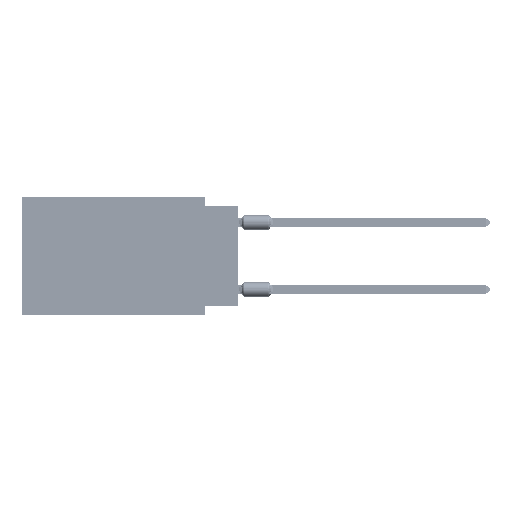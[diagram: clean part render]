
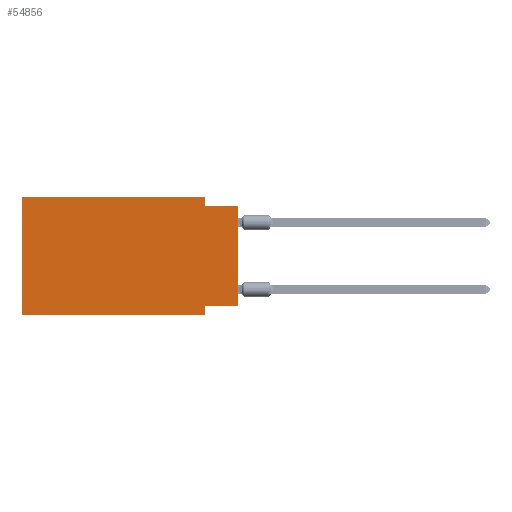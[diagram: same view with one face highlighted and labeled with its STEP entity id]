
A CAD part, left-side view. The second image highlights one B-rep face of the part: STEP entity #54856.
In plain terms, the highlighted planar face has unit normal (-1, 0, 0).
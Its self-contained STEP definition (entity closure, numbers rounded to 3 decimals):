
#1090 = VERTEX_POINT ( 'NONE', #2675 ) ;
#2675 = CARTESIAN_POINT ( 'NONE',  ( 0., 0., -0.635 ) ) ;
#5478 = EDGE_CURVE ( 'NONE', #78072, #86464, #22740, .T. ) ;
#10530 = LINE ( 'NONE', #24280, #24152 ) ;
#12280 = DIRECTION ( 'NONE',  ( 0., 0., -1. ) ) ;
#12432 = PLANE ( 'NONE',  #39319 ) ;
#13697 = CARTESIAN_POINT ( 'NONE',  ( 0., 16.383, 0. ) ) ;
#14303 = EDGE_LOOP ( 'NONE', ( #94507, #85639, #62938, #16057, #21806, #57369, #17778, #51122 ) ) ;
#15489 = LINE ( 'NONE', #13697, #29186 ) ;
#16057 = ORIENTED_EDGE ( 'NONE', *, *, #51140, .F. ) ;
#16251 = CARTESIAN_POINT ( 'NONE',  ( 0., 2.54, -8.89 ) ) ;
#17050 = VECTOR ( 'NONE', #87482, 1000. ) ;
#17396 = CARTESIAN_POINT ( 'NONE',  ( 0., 16.383, -8.89 ) ) ;
#17778 = ORIENTED_EDGE ( 'NONE', *, *, #53410, .F. ) ;
#19549 = CARTESIAN_POINT ( 'NONE',  ( 0., 0., -8.255 ) ) ;
#20548 = VERTEX_POINT ( 'NONE', #93034 ) ;
#21164 = VERTEX_POINT ( 'NONE', #45767 ) ;
#21294 = CARTESIAN_POINT ( 'NONE',  ( 0., 16.383, 0. ) ) ;
#21304 = VECTOR ( 'NONE', #44368, 1000. ) ;
#21806 = ORIENTED_EDGE ( 'NONE', *, *, #5478, .F. ) ;
#22740 = LINE ( 'NONE', #21294, #21304 ) ;
#23143 = LINE ( 'NONE', #16251, #23464 ) ;
#23371 = CARTESIAN_POINT ( 'NONE',  ( 0., 0., -8.255 ) ) ;
#23464 = VECTOR ( 'NONE', #46205, 1000. ) ;
#24152 = VECTOR ( 'NONE', #40495, 1000. ) ;
#24280 = CARTESIAN_POINT ( 'NONE',  ( 0., 0., -0.635 ) ) ;
#25070 = LINE ( 'NONE', #85892, #81074 ) ;
#26022 = VECTOR ( 'NONE', #60799, 1000. ) ;
#26183 = DIRECTION ( 'NONE',  ( 1., 0., 0. ) ) ;
#26671 = DIRECTION ( 'NONE',  ( 0., 0., -1. ) ) ;
#29186 = VECTOR ( 'NONE', #35810, 1000. ) ;
#30837 = EDGE_CURVE ( 'NONE', #20548, #40981, #25070, .T. ) ;
#30853 = LINE ( 'NONE', #68627, #26022 ) ;
#31226 = DIRECTION ( 'NONE',  ( 0., 1., 0. ) ) ;
#35810 = DIRECTION ( 'NONE',  ( 0., -1., 0. ) ) ;
#39168 = VERTEX_POINT ( 'NONE', #55024 ) ;
#39319 = AXIS2_PLACEMENT_3D ( 'NONE', #49263, #26183, #26671 ) ;
#39852 = EDGE_CURVE ( 'NONE', #67837, #21164, #74428, .T. ) ;
#40495 = DIRECTION ( 'NONE',  ( 0., -1., 0. ) ) ;
#40561 = VECTOR ( 'NONE', #31226, 1000. ) ;
#40981 = VERTEX_POINT ( 'NONE', #73010 ) ;
#41421 = FACE_OUTER_BOUND ( 'NONE', #14303, .T. ) ;
#41853 = EDGE_CURVE ( 'NONE', #78072, #39168, #72787, .T. ) ;
#44368 = DIRECTION ( 'NONE',  ( 0., 0., 1. ) ) ;
#45767 = CARTESIAN_POINT ( 'NONE',  ( 0., 2.54, -8.255 ) ) ;
#46205 = DIRECTION ( 'NONE',  ( 0., 0., -1. ) ) ;
#49263 = CARTESIAN_POINT ( 'NONE',  ( 0., 16.383, 0. ) ) ;
#51122 = ORIENTED_EDGE ( 'NONE', *, *, #39852, .F. ) ;
#51140 = EDGE_CURVE ( 'NONE', #86464, #20548, #15489, .T. ) ;
#53410 = EDGE_CURVE ( 'NONE', #21164, #39168, #23143, .T. ) ;
#54856 = ADVANCED_FACE ( 'NONE', ( #41421 ), #12432, .F. ) ;
#55024 = CARTESIAN_POINT ( 'NONE',  ( 0., 2.54, -8.89 ) ) ;
#57369 = ORIENTED_EDGE ( 'NONE', *, *, #41853, .T. ) ;
#60799 = DIRECTION ( 'NONE',  ( 0., 0., 1. ) ) ;
#62938 = ORIENTED_EDGE ( 'NONE', *, *, #30837, .F. ) ;
#67837 = VERTEX_POINT ( 'NONE', #19549 ) ;
#68580 = CARTESIAN_POINT ( 'NONE',  ( 0., 16.383, 0. ) ) ;
#68627 = CARTESIAN_POINT ( 'NONE',  ( 0., 0., 0. ) ) ;
#72787 = LINE ( 'NONE', #93861, #17050 ) ;
#73010 = CARTESIAN_POINT ( 'NONE',  ( 0., 2.54, -0.635 ) ) ;
#74428 = LINE ( 'NONE', #23371, #40561 ) ;
#77844 = EDGE_CURVE ( 'NONE', #67837, #1090, #30853, .T. ) ;
#78072 = VERTEX_POINT ( 'NONE', #17396 ) ;
#81074 = VECTOR ( 'NONE', #12280, 1000. ) ;
#82553 = EDGE_CURVE ( 'NONE', #40981, #1090, #10530, .T. ) ;
#85639 = ORIENTED_EDGE ( 'NONE', *, *, #82553, .F. ) ;
#85892 = CARTESIAN_POINT ( 'NONE',  ( 0., 2.54, 0. ) ) ;
#86464 = VERTEX_POINT ( 'NONE', #68580 ) ;
#87482 = DIRECTION ( 'NONE',  ( 0., -1., 0. ) ) ;
#93034 = CARTESIAN_POINT ( 'NONE',  ( 0., 2.54, 0. ) ) ;
#93861 = CARTESIAN_POINT ( 'NONE',  ( 0., 16.383, -8.89 ) ) ;
#94507 = ORIENTED_EDGE ( 'NONE', *, *, #77844, .T. ) ;
